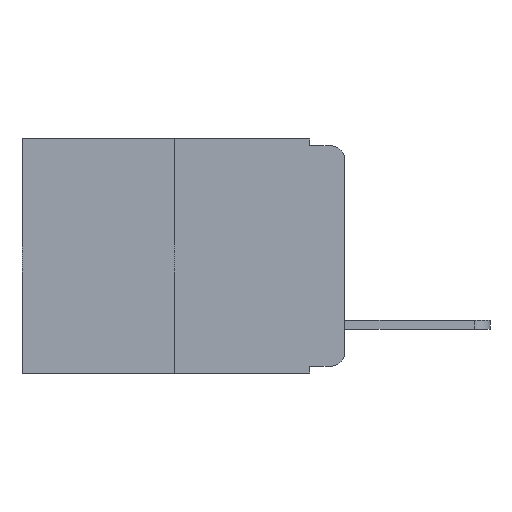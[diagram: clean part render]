
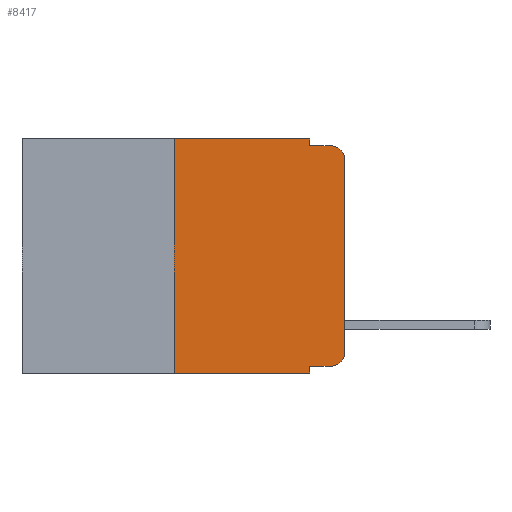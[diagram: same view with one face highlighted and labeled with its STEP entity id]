
A CAD part, left-side view. The second image highlights one B-rep face of the part: STEP entity #8417.
In plain terms, the highlighted planar face has unit normal (-1, 0, 0).
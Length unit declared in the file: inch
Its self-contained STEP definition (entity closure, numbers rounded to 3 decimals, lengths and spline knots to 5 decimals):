
#268 = DIRECTION ( 'NONE',  ( 0., 0., -1. ) ) ;
#356 = VECTOR ( 'NONE', #6270, 39.37008 ) ;
#641 = VERTEX_POINT ( 'NONE', #6732 ) ;
#801 = VECTOR ( 'NONE', #11022, 39.37008 ) ;
#1116 = LINE ( 'NONE', #6668, #801 ) ;
#1137 = CARTESIAN_POINT ( 'NONE',  ( 0., 0.051, -0.01 ) ) ;
#1800 = CARTESIAN_POINT ( 'NONE',  ( 0., 0.051, -0.333 ) ) ;
#1889 = EDGE_CURVE ( 'NONE', #12076, #8148, #10290, .T. ) ;
#2102 = CARTESIAN_POINT ( 'NONE',  ( 0., 0., 0. ) ) ;
#2116 = EDGE_LOOP ( 'NONE', ( #8612, #7246, #7110, #6205, #5933, #3970, #2909, #7192, #7309, #7902 ) ) ;
#2478 = CARTESIAN_POINT ( 'NONE',  ( 0., 0.02, -0.313 ) ) ;
#2479 = CARTESIAN_POINT ( 'NONE',  ( 0., 0.25, 0. ) ) ;
#2909 = ORIENTED_EDGE ( 'NONE', *, *, #1889, .T. ) ;
#3046 = LINE ( 'NONE', #1137, #5278 ) ;
#3260 = DIRECTION ( 'NONE',  ( 0., 0., 1. ) ) ;
#3264 = DIRECTION ( 'NONE',  ( -1., 0., 0. ) ) ;
#3296 = EDGE_CURVE ( 'NONE', #641, #12215, #9230, .T. ) ;
#3337 = VECTOR ( 'NONE', #3260, 39.37008 ) ;
#3947 = CIRCLE ( 'NONE', #9261, 0.02 ) ;
#3970 = ORIENTED_EDGE ( 'NONE', *, *, #9745, .F. ) ;
#4217 = CARTESIAN_POINT ( 'NONE',  ( 0., 0.25, 0. ) ) ;
#4292 = CARTESIAN_POINT ( 'NONE',  ( 0., 0.25, -0.343 ) ) ;
#4334 = DIRECTION ( 'NONE',  ( 0., 0., -1. ) ) ;
#4518 = VECTOR ( 'NONE', #10873, 39.37008 ) ;
#4758 = VERTEX_POINT ( 'NONE', #10791 ) ;
#5010 = LINE ( 'NONE', #2102, #10092 ) ;
#5012 = VERTEX_POINT ( 'NONE', #6644 ) ;
#5048 = DIRECTION ( 'NONE',  ( 1., 0., 0. ) ) ;
#5073 = PLANE ( 'NONE',  #6563 ) ;
#5234 = VECTOR ( 'NONE', #11123, 39.37008 ) ;
#5278 = VECTOR ( 'NONE', #6761, 39.37008 ) ;
#5355 = VERTEX_POINT ( 'NONE', #11052 ) ;
#5518 = LINE ( 'NONE', #9273, #5234 ) ;
#5724 = EDGE_CURVE ( 'NONE', #12215, #5355, #5010, .T. ) ;
#5933 = ORIENTED_EDGE ( 'NONE', *, *, #7193, .F. ) ;
#5955 = CARTESIAN_POINT ( 'NONE',  ( 0., 0.473, 0. ) ) ;
#6174 = VERTEX_POINT ( 'NONE', #1800 ) ;
#6195 = CARTESIAN_POINT ( 'NONE',  ( 0., 0.473, -0.343 ) ) ;
#6205 = ORIENTED_EDGE ( 'NONE', *, *, #9414, .F. ) ;
#6270 = DIRECTION ( 'NONE',  ( 0., -1., 0. ) ) ;
#6531 = DIRECTION ( 'NONE',  ( -1., 0., 0. ) ) ;
#6563 = AXIS2_PLACEMENT_3D ( 'NONE', #5955, #5048, #4334 ) ;
#6589 = DIRECTION ( 'NONE',  ( 0., -1., 0. ) ) ;
#6644 = CARTESIAN_POINT ( 'NONE',  ( 0., 0.051, -0.01 ) ) ;
#6668 = CARTESIAN_POINT ( 'NONE',  ( 0., 0.051, -0.333 ) ) ;
#6732 = CARTESIAN_POINT ( 'NONE',  ( 0., 0.02, -0.333 ) ) ;
#6761 = DIRECTION ( 'NONE',  ( 0., -1., 0. ) ) ;
#7075 = VERTEX_POINT ( 'NONE', #8116 ) ;
#7110 = ORIENTED_EDGE ( 'NONE', *, *, #9151, .F. ) ;
#7192 = ORIENTED_EDGE ( 'NONE', *, *, #10938, .F. ) ;
#7193 = EDGE_CURVE ( 'NONE', #8112, #7075, #10655, .T. ) ;
#7246 = ORIENTED_EDGE ( 'NONE', *, *, #9508, .T. ) ;
#7309 = ORIENTED_EDGE ( 'NONE', *, *, #11066, .T. ) ;
#7489 = FACE_OUTER_BOUND ( 'NONE', #2116, .T. ) ;
#7802 = CARTESIAN_POINT ( 'NONE',  ( 0., 0., -0.313 ) ) ;
#7902 = ORIENTED_EDGE ( 'NONE', *, *, #3296, .T. ) ;
#8112 = VERTEX_POINT ( 'NONE', #2479 ) ;
#8116 = CARTESIAN_POINT ( 'NONE',  ( 0., 0.051, 0. ) ) ;
#8148 = VERTEX_POINT ( 'NONE', #10229 ) ;
#8417 = ADVANCED_FACE ( 'NONE', ( #7489 ), #5073, .F. ) ;
#8612 = ORIENTED_EDGE ( 'NONE', *, *, #5724, .T. ) ;
#9151 = EDGE_CURVE ( 'NONE', #5012, #4758, #3046, .T. ) ;
#9230 = CIRCLE ( 'NONE', #10096, 0.02 ) ;
#9261 = AXIS2_PLACEMENT_3D ( 'NONE', #12043, #6531, #10349 ) ;
#9273 = CARTESIAN_POINT ( 'NONE',  ( 0., 0.051, 0. ) ) ;
#9414 = EDGE_CURVE ( 'NONE', #7075, #5012, #11925, .T. ) ;
#9508 = EDGE_CURVE ( 'NONE', #5355, #4758, #3947, .T. ) ;
#9745 = EDGE_CURVE ( 'NONE', #12076, #8112, #11126, .T. ) ;
#9984 = CARTESIAN_POINT ( 'NONE',  ( 0., 0.051, 0. ) ) ;
#10092 = VECTOR ( 'NONE', #11208, 39.37008 ) ;
#10096 = AXIS2_PLACEMENT_3D ( 'NONE', #2478, #3264, #268 ) ;
#10229 = CARTESIAN_POINT ( 'NONE',  ( 0., 0.051, -0.343 ) ) ;
#10290 = LINE ( 'NONE', #6195, #356 ) ;
#10349 = DIRECTION ( 'NONE',  ( 0., 0., -1. ) ) ;
#10374 = VECTOR ( 'NONE', #6589, 39.37008 ) ;
#10655 = LINE ( 'NONE', #11024, #10374 ) ;
#10791 = CARTESIAN_POINT ( 'NONE',  ( 0., 0.02, -0.01 ) ) ;
#10873 = DIRECTION ( 'NONE',  ( 0., 0., -1. ) ) ;
#10938 = EDGE_CURVE ( 'NONE', #6174, #8148, #5518, .T. ) ;
#11022 = DIRECTION ( 'NONE',  ( 0., -1., 0. ) ) ;
#11024 = CARTESIAN_POINT ( 'NONE',  ( 0., 0.473, 0. ) ) ;
#11052 = CARTESIAN_POINT ( 'NONE',  ( 0., 0., -0.03 ) ) ;
#11066 = EDGE_CURVE ( 'NONE', #6174, #641, #1116, .T. ) ;
#11123 = DIRECTION ( 'NONE',  ( 0., 0., -1. ) ) ;
#11126 = LINE ( 'NONE', #4217, #3337 ) ;
#11208 = DIRECTION ( 'NONE',  ( 0., 0., 1. ) ) ;
#11925 = LINE ( 'NONE', #9984, #4518 ) ;
#12043 = CARTESIAN_POINT ( 'NONE',  ( 0., 0.02, -0.03 ) ) ;
#12076 = VERTEX_POINT ( 'NONE', #4292 ) ;
#12215 = VERTEX_POINT ( 'NONE', #7802 ) ;
